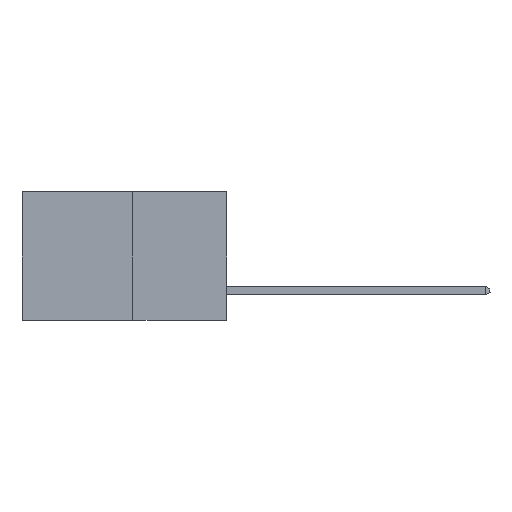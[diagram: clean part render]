
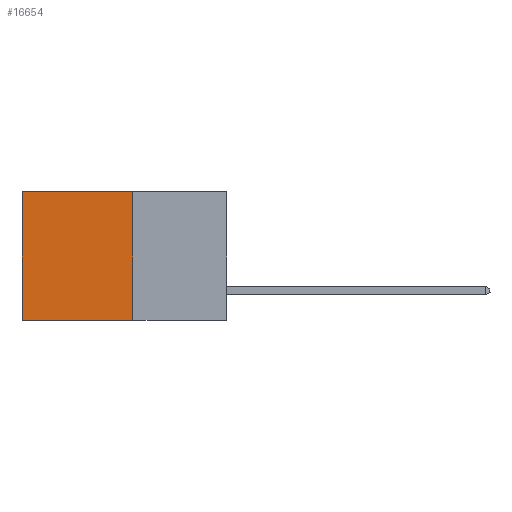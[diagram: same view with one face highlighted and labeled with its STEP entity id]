
A CAD part, left-side view. The second image highlights one B-rep face of the part: STEP entity #16654.
In plain terms, the highlighted planar face has unit normal (-1, 0, 0).
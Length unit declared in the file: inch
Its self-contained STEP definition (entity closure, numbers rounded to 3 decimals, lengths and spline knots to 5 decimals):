
#62 = ORIENTED_EDGE ( 'NONE', *, *, #23309, .T. ) ;
#1385 = LINE ( 'NONE', #18511, #22527 ) ;
#1900 = LINE ( 'NONE', #10762, #18181 ) ;
#2202 = ORIENTED_EDGE ( 'NONE', *, *, #11822, .F. ) ;
#2717 = CARTESIAN_POINT ( 'NONE',  ( 0.277, 0.59, -0.37 ) ) ;
#5310 = LINE ( 'NONE', #8884, #21486 ) ;
#6497 = CARTESIAN_POINT ( 'NONE',  ( 0.277, 0.27, -0.37 ) ) ;
#6614 = ORIENTED_EDGE ( 'NONE', *, *, #22258, .T. ) ;
#7429 = FACE_OUTER_BOUND ( 'NONE', #10121, .T. ) ;
#7991 = CARTESIAN_POINT ( 'NONE',  ( 0.277, 0.27, -0.37 ) ) ;
#8250 = VERTEX_POINT ( 'NONE', #15332 ) ;
#8632 = VERTEX_POINT ( 'NONE', #26924 ) ;
#8884 = CARTESIAN_POINT ( 'NONE',  ( 0.277, 0.59, -0.37 ) ) ;
#10112 = DIRECTION ( 'NONE',  ( 0., 0., -1. ) ) ;
#10121 = EDGE_LOOP ( 'NONE', ( #62, #2202, #11662, #6614 ) ) ;
#10762 = CARTESIAN_POINT ( 'NONE',  ( 0.277, 0.27, -0.37 ) ) ;
#11662 = ORIENTED_EDGE ( 'NONE', *, *, #26973, .F. ) ;
#11822 = EDGE_CURVE ( 'NONE', #8632, #22635, #20797, .T. ) ;
#12071 = CARTESIAN_POINT ( 'NONE',  ( 0.277, 0.59, 0. ) ) ;
#12833 = DIRECTION ( 'NONE',  ( 0., 0., -1. ) ) ;
#14231 = PLANE ( 'NONE',  #22976 ) ;
#15332 = CARTESIAN_POINT ( 'NONE',  ( 0.277, 0.27, 0. ) ) ;
#15393 = VERTEX_POINT ( 'NONE', #12071 ) ;
#16654 = ADVANCED_FACE ( 'NONE', ( #7429 ), #14231, .F. ) ;
#18181 = VECTOR ( 'NONE', #12833, 39.37008 ) ;
#18511 = CARTESIAN_POINT ( 'NONE',  ( 0.277, 0.27, 0. ) ) ;
#19446 = DIRECTION ( 'NONE',  ( 0., 0., -1. ) ) ;
#20599 = DIRECTION ( 'NONE',  ( 0., 1., 0. ) ) ;
#20797 = LINE ( 'NONE', #6497, #21431 ) ;
#21236 = DIRECTION ( 'NONE',  ( 0., 1., 0. ) ) ;
#21431 = VECTOR ( 'NONE', #21236, 39.37008 ) ;
#21486 = VECTOR ( 'NONE', #19446, 39.37008 ) ;
#22258 = EDGE_CURVE ( 'NONE', #8250, #15393, #1385, .T. ) ;
#22527 = VECTOR ( 'NONE', #20599, 39.37008 ) ;
#22635 = VERTEX_POINT ( 'NONE', #2717 ) ;
#22689 = DIRECTION ( 'NONE',  ( 1., 0., 0. ) ) ;
#22976 = AXIS2_PLACEMENT_3D ( 'NONE', #7991, #22689, #10112 ) ;
#23309 = EDGE_CURVE ( 'NONE', #15393, #22635, #5310, .T. ) ;
#26924 = CARTESIAN_POINT ( 'NONE',  ( 0.277, 0.27, -0.37 ) ) ;
#26973 = EDGE_CURVE ( 'NONE', #8250, #8632, #1900, .T. ) ;
